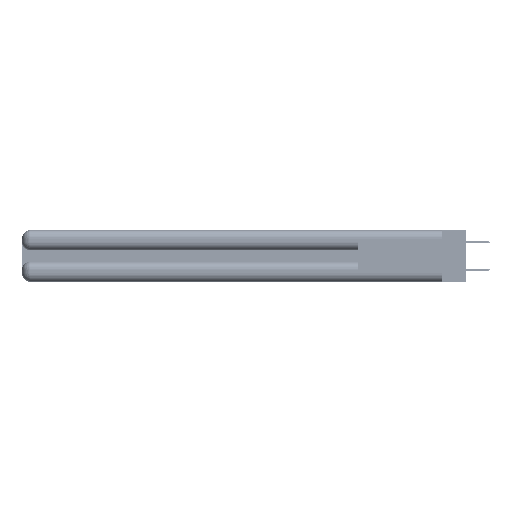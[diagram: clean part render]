
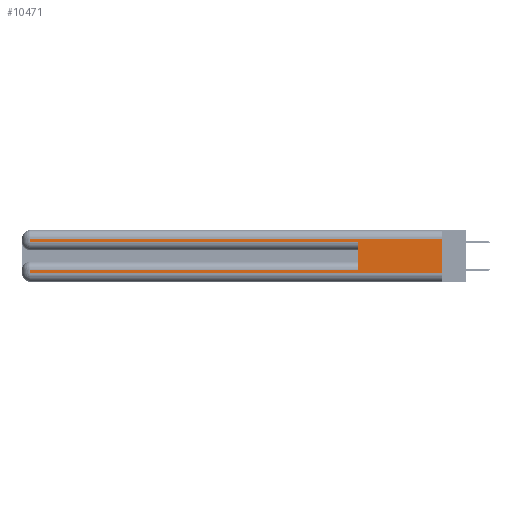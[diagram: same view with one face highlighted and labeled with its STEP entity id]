
A CAD part, left-side view. The second image highlights one B-rep face of the part: STEP entity #10471.
In plain terms, the highlighted planar face has unit normal (-1, 0, 0).
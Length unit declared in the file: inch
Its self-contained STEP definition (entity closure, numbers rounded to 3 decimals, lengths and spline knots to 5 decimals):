
#2776 = VECTOR ( 'NONE', #49577, 39.37008 ) ;
#2783 = DIRECTION ( 'NONE',  ( 0., 0., 1. ) ) ;
#3111 = PLANE ( 'NONE',  #14479 ) ;
#4034 = LINE ( 'NONE', #45547, #2776 ) ;
#5100 = CARTESIAN_POINT ( 'NONE',  ( 0., 2.94, 0.31 ) ) ;
#5259 = EDGE_CURVE ( 'NONE', #12359, #37839, #31964, .T. ) ;
#5774 = CARTESIAN_POINT ( 'NONE',  ( 0., 0.6, 0.285 ) ) ;
#6222 = DIRECTION ( 'NONE',  ( 0., 0., -1. ) ) ;
#6691 = CARTESIAN_POINT ( 'NONE',  ( 0., 0.6, 0.145 ) ) ;
#7172 = DIRECTION ( 'NONE',  ( 1., 0., 0. ) ) ;
#7497 = CARTESIAN_POINT ( 'NONE',  ( 0., 0., 0.31 ) ) ;
#10471 = ADVANCED_FACE ( 'NONE', ( #11537 ), #3111, .F. ) ;
#11480 = VECTOR ( 'NONE', #31890, 39.37008 ) ;
#11537 = FACE_OUTER_BOUND ( 'NONE', #50237, .T. ) ;
#12293 = CARTESIAN_POINT ( 'NONE',  ( 0., 0.6, 0.085 ) ) ;
#12359 = VERTEX_POINT ( 'NONE', #12293 ) ;
#14479 = AXIS2_PLACEMENT_3D ( 'NONE', #15127, #7172, #35337 ) ;
#14566 = LINE ( 'NONE', #47673, #35943 ) ;
#14737 = CARTESIAN_POINT ( 'NONE',  ( 0., 0., 0.06 ) ) ;
#14858 = EDGE_CURVE ( 'NONE', #36684, #31324, #4034, .T. ) ;
#14975 = ORIENTED_EDGE ( 'NONE', *, *, #20030, .T. ) ;
#15127 = CARTESIAN_POINT ( 'NONE',  ( 0., 0., 0.37 ) ) ;
#15511 = LINE ( 'NONE', #46504, #26328 ) ;
#15950 = ORIENTED_EDGE ( 'NONE', *, *, #32020, .F. ) ;
#19682 = LINE ( 'NONE', #46255, #29137 ) ;
#20030 = EDGE_CURVE ( 'NONE', #51188, #23688, #15511, .T. ) ;
#20752 = CARTESIAN_POINT ( 'NONE',  ( 0., 2.94, 0.085 ) ) ;
#23688 = VERTEX_POINT ( 'NONE', #5100 ) ;
#24379 = VERTEX_POINT ( 'NONE', #45993 ) ;
#26328 = VECTOR ( 'NONE', #50524, 39.37008 ) ;
#26733 = EDGE_CURVE ( 'NONE', #37839, #24379, #14566, .T. ) ;
#26797 = DIRECTION ( 'NONE',  ( 0., -1., 0. ) ) ;
#29137 = VECTOR ( 'NONE', #6222, 39.37008 ) ;
#30172 = VECTOR ( 'NONE', #26797, 39.37008 ) ;
#30367 = CARTESIAN_POINT ( 'NONE',  ( 0., 2.94, 0.285 ) ) ;
#30520 = VECTOR ( 'NONE', #2783, 39.37008 ) ;
#30824 = EDGE_CURVE ( 'NONE', #12359, #31324, #42397, .T. ) ;
#31200 = VERTEX_POINT ( 'NONE', #33050 ) ;
#31319 = ORIENTED_EDGE ( 'NONE', *, *, #43953, .T. ) ;
#31324 = VERTEX_POINT ( 'NONE', #5774 ) ;
#31890 = DIRECTION ( 'NONE',  ( 0., 0., -1. ) ) ;
#31964 = LINE ( 'NONE', #40886, #42623 ) ;
#32020 = EDGE_CURVE ( 'NONE', #51188, #31200, #19682, .T. ) ;
#32565 = ORIENTED_EDGE ( 'NONE', *, *, #26733, .T. ) ;
#33050 = CARTESIAN_POINT ( 'NONE',  ( 0., 0., 0.06 ) ) ;
#35337 = DIRECTION ( 'NONE',  ( 0., 0., -1. ) ) ;
#35825 = DIRECTION ( 'NONE',  ( 0., 0., -1. ) ) ;
#35943 = VECTOR ( 'NONE', #35825, 39.37008 ) ;
#36478 = ORIENTED_EDGE ( 'NONE', *, *, #14858, .T. ) ;
#36684 = VERTEX_POINT ( 'NONE', #30367 ) ;
#37839 = VERTEX_POINT ( 'NONE', #20752 ) ;
#40886 = CARTESIAN_POINT ( 'NONE',  ( 0., 0., 0.085 ) ) ;
#42397 = LINE ( 'NONE', #6691, #30520 ) ;
#42623 = VECTOR ( 'NONE', #44899, 39.37008 ) ;
#43568 = LINE ( 'NONE', #51801, #11480 ) ;
#43953 = EDGE_CURVE ( 'NONE', #23688, #36684, #43568, .T. ) ;
#44019 = ORIENTED_EDGE ( 'NONE', *, *, #48552, .T. ) ;
#44899 = DIRECTION ( 'NONE',  ( 0., 1., 0. ) ) ;
#45547 = CARTESIAN_POINT ( 'NONE',  ( 0., 0., 0.285 ) ) ;
#45587 = ORIENTED_EDGE ( 'NONE', *, *, #5259, .T. ) ;
#45993 = CARTESIAN_POINT ( 'NONE',  ( 0., 2.94, 0.06 ) ) ;
#46255 = CARTESIAN_POINT ( 'NONE',  ( 0., 0., 0.37 ) ) ;
#46504 = CARTESIAN_POINT ( 'NONE',  ( 0., 0., 0.31 ) ) ;
#47673 = CARTESIAN_POINT ( 'NONE',  ( 0., 2.94, 0.37 ) ) ;
#48187 = ORIENTED_EDGE ( 'NONE', *, *, #30824, .F. ) ;
#48552 = EDGE_CURVE ( 'NONE', #24379, #31200, #51391, .T. ) ;
#49577 = DIRECTION ( 'NONE',  ( 0., -1., 0. ) ) ;
#50237 = EDGE_LOOP ( 'NONE', ( #15950, #14975, #31319, #36478, #48187, #45587, #32565, #44019 ) ) ;
#50524 = DIRECTION ( 'NONE',  ( 0., 1., 0. ) ) ;
#51188 = VERTEX_POINT ( 'NONE', #7497 ) ;
#51391 = LINE ( 'NONE', #14737, #30172 ) ;
#51801 = CARTESIAN_POINT ( 'NONE',  ( 0., 2.94, 0.37 ) ) ;
